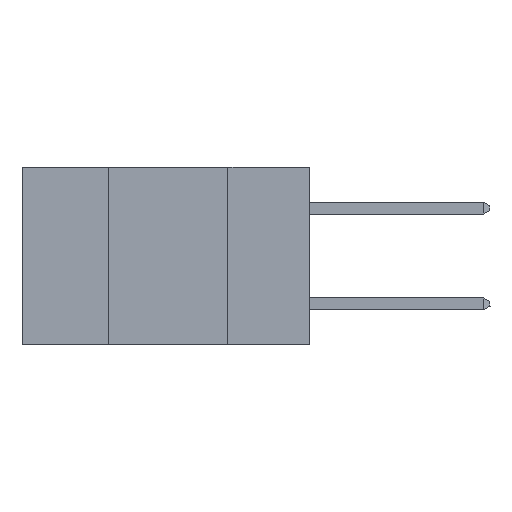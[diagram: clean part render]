
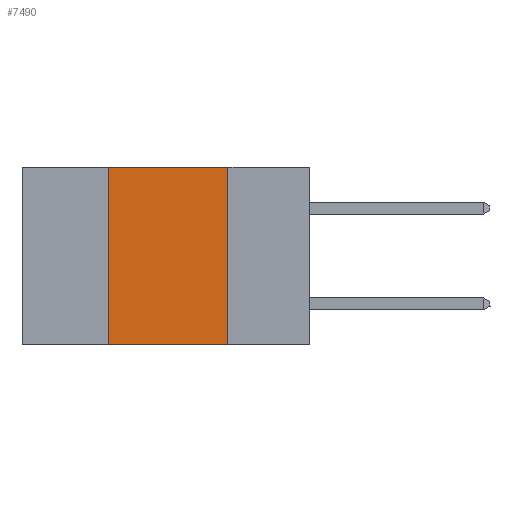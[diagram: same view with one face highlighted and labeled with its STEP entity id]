
A CAD part, left-side view. The second image highlights one B-rep face of the part: STEP entity #7490.
In plain terms, the highlighted planar face has unit normal (-1, 0, 0).
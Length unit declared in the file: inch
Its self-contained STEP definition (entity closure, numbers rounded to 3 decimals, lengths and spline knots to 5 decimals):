
#508 = VERTEX_POINT ( 'NONE', #34206 ) ;
#2086 = CARTESIAN_POINT ( 'NONE',  ( 0., 0.6, 0. ) ) ;
#2538 = VECTOR ( 'NONE', #12603, 39.37008 ) ;
#2684 = VECTOR ( 'NONE', #5547, 39.37008 ) ;
#2856 = FACE_OUTER_BOUND ( 'NONE', #31162, .T. ) ;
#3534 = LINE ( 'NONE', #21881, #2684 ) ;
#4618 = LINE ( 'NONE', #7060, #7636 ) ;
#5547 = DIRECTION ( 'NONE',  ( 0., 0., -1. ) ) ;
#5876 = PLANE ( 'NONE',  #7956 ) ;
#5962 = VERTEX_POINT ( 'NONE', #10667 ) ;
#5992 = CARTESIAN_POINT ( 'NONE',  ( 0., 0.6, 0. ) ) ;
#7060 = CARTESIAN_POINT ( 'NONE',  ( 0., 0.6, -0.37 ) ) ;
#7490 = ADVANCED_FACE ( 'NONE', ( #2856 ), #5876, .F. ) ;
#7618 = VERTEX_POINT ( 'NONE', #24527 ) ;
#7636 = VECTOR ( 'NONE', #20825, 39.37008 ) ;
#7956 = AXIS2_PLACEMENT_3D ( 'NONE', #5992, #24983, #8408 ) ;
#8408 = DIRECTION ( 'NONE',  ( 0., 0., -1. ) ) ;
#10667 = CARTESIAN_POINT ( 'NONE',  ( 0., 0.17, -0.37 ) ) ;
#12603 = DIRECTION ( 'NONE',  ( 0., 0., 1. ) ) ;
#13138 = DIRECTION ( 'NONE',  ( 0., -1., 0. ) ) ;
#14319 = ORIENTED_EDGE ( 'NONE', *, *, #20286, .F. ) ;
#16143 = EDGE_CURVE ( 'NONE', #28523, #5962, #3534, .T. ) ;
#18601 = ORIENTED_EDGE ( 'NONE', *, *, #26653, .F. ) ;
#20257 = VECTOR ( 'NONE', #13138, 39.37008 ) ;
#20286 = EDGE_CURVE ( 'NONE', #508, #7618, #31456, .T. ) ;
#20825 = DIRECTION ( 'NONE',  ( 0., -1., 0. ) ) ;
#21881 = CARTESIAN_POINT ( 'NONE',  ( 0., 0.17, 0. ) ) ;
#24527 = CARTESIAN_POINT ( 'NONE',  ( 0., 0.42, 0. ) ) ;
#24983 = DIRECTION ( 'NONE',  ( 1., 0., 0. ) ) ;
#25307 = CARTESIAN_POINT ( 'NONE',  ( 0., 0.17, 0. ) ) ;
#26653 = EDGE_CURVE ( 'NONE', #7618, #28523, #30189, .T. ) ;
#28523 = VERTEX_POINT ( 'NONE', #25307 ) ;
#28938 = CARTESIAN_POINT ( 'NONE',  ( 0., 0.42, 0. ) ) ;
#30189 = LINE ( 'NONE', #2086, #20257 ) ;
#31162 = EDGE_LOOP ( 'NONE', ( #31192, #18601, #14319, #31883 ) ) ;
#31192 = ORIENTED_EDGE ( 'NONE', *, *, #16143, .F. ) ;
#31456 = LINE ( 'NONE', #28938, #2538 ) ;
#31883 = ORIENTED_EDGE ( 'NONE', *, *, #34682, .T. ) ;
#34206 = CARTESIAN_POINT ( 'NONE',  ( 0., 0.42, -0.37 ) ) ;
#34682 = EDGE_CURVE ( 'NONE', #508, #5962, #4618, .T. ) ;
